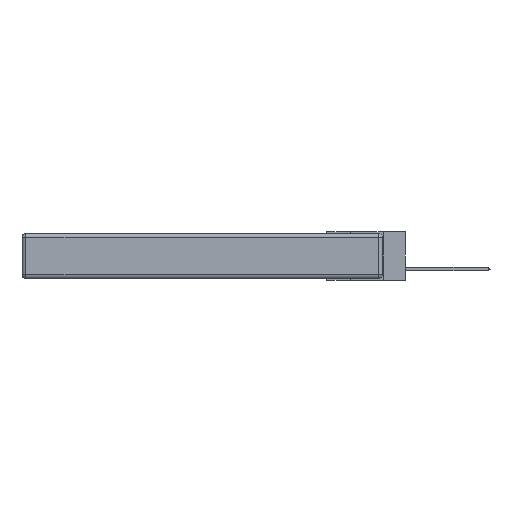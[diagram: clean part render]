
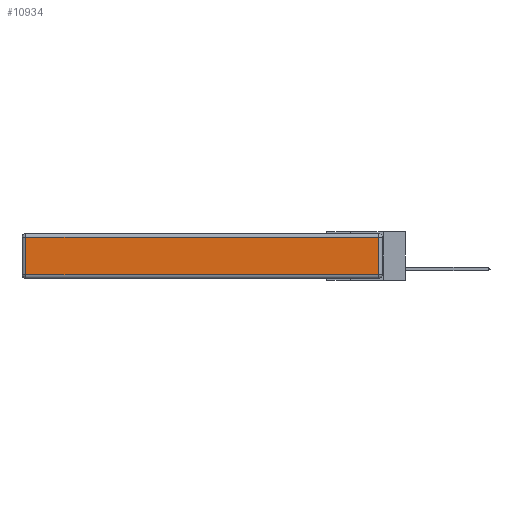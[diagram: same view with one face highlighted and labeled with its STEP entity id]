
A CAD part, left-side view. The second image highlights one B-rep face of the part: STEP entity #10934.
In plain terms, the highlighted planar face has unit normal (-1, 0, 0).
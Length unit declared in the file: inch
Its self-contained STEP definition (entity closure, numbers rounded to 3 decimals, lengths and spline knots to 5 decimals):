
#86 = VERTEX_POINT ( 'NONE', #7039 ) ;
#342 = DIRECTION ( 'NONE',  ( 0., 0., 1. ) ) ;
#529 = CARTESIAN_POINT ( 'NONE',  ( 0., 2.72, -0.313 ) ) ;
#1624 = ORIENTED_EDGE ( 'NONE', *, *, #2034, .T. ) ;
#2034 = EDGE_CURVE ( 'NONE', #5893, #86, #10985, .T. ) ;
#2467 = CARTESIAN_POINT ( 'NONE',  ( 0., 2.75, -0.03 ) ) ;
#3245 = ORIENTED_EDGE ( 'NONE', *, *, #9848, .T. ) ;
#3428 = VERTEX_POINT ( 'NONE', #7598 ) ;
#4119 = CARTESIAN_POINT ( 'NONE',  ( 0., 0.03, -0.343 ) ) ;
#4556 = DIRECTION ( 'NONE',  ( -1., 0., 0. ) ) ;
#4981 = VECTOR ( 'NONE', #7885, 39.37008 ) ;
#5434 = CARTESIAN_POINT ( 'NONE',  ( 0., 2.72, -0.03 ) ) ;
#5646 = LINE ( 'NONE', #2467, #4981 ) ;
#5734 = ORIENTED_EDGE ( 'NONE', *, *, #7126, .T. ) ;
#5893 = VERTEX_POINT ( 'NONE', #529 ) ;
#6163 = ORIENTED_EDGE ( 'NONE', *, *, #11180, .T. ) ;
#6534 = CARTESIAN_POINT ( 'NONE',  ( 0., 2.72, -0.343 ) ) ;
#7039 = CARTESIAN_POINT ( 'NONE',  ( 0., 0.03, -0.313 ) ) ;
#7126 = EDGE_CURVE ( 'NONE', #86, #3428, #8745, .T. ) ;
#7598 = CARTESIAN_POINT ( 'NONE',  ( 0., 0.03, -0.03 ) ) ;
#7885 = DIRECTION ( 'NONE',  ( 0., 1., 0. ) ) ;
#8484 = VECTOR ( 'NONE', #12813, 39.37008 ) ;
#8745 = LINE ( 'NONE', #4119, #12595 ) ;
#8844 = VECTOR ( 'NONE', #9748, 39.37008 ) ;
#9018 = CARTESIAN_POINT ( 'NONE',  ( 0., 0., -0.343 ) ) ;
#9516 = FACE_OUTER_BOUND ( 'NONE', #9807, .T. ) ;
#9696 = CARTESIAN_POINT ( 'NONE',  ( 0., 0., -0.313 ) ) ;
#9748 = DIRECTION ( 'NONE',  ( 0., 0., -1. ) ) ;
#9807 = EDGE_LOOP ( 'NONE', ( #1624, #5734, #6163, #3245 ) ) ;
#9809 = AXIS2_PLACEMENT_3D ( 'NONE', #9018, #4556, #342 ) ;
#9848 = EDGE_CURVE ( 'NONE', #10814, #5893, #9877, .T. ) ;
#9877 = LINE ( 'NONE', #6534, #8844 ) ;
#10814 = VERTEX_POINT ( 'NONE', #5434 ) ;
#10934 = ADVANCED_FACE ( 'NONE', ( #9516 ), #13138, .T. ) ;
#10985 = LINE ( 'NONE', #9696, #8484 ) ;
#11180 = EDGE_CURVE ( 'NONE', #3428, #10814, #5646, .T. ) ;
#12595 = VECTOR ( 'NONE', #12667, 39.37008 ) ;
#12667 = DIRECTION ( 'NONE',  ( 0., 0., 1. ) ) ;
#12813 = DIRECTION ( 'NONE',  ( 0., -1., 0. ) ) ;
#13138 = PLANE ( 'NONE',  #9809 ) ;
